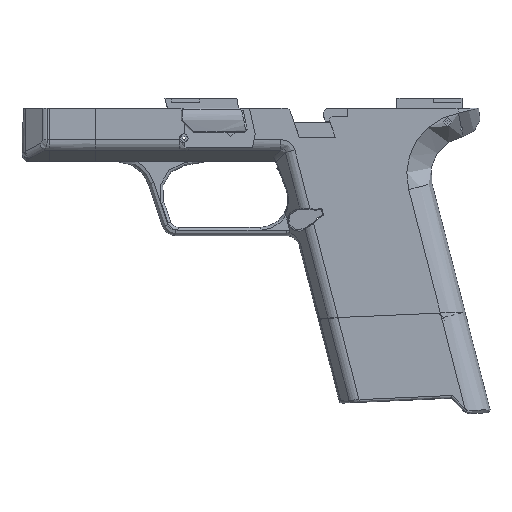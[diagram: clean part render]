
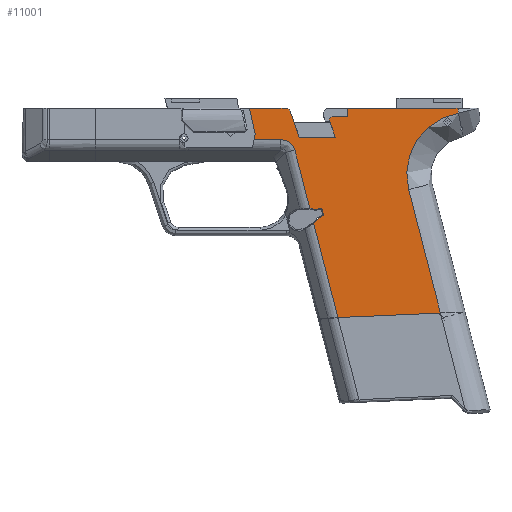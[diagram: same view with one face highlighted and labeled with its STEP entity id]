
A CAD part, left-side view. The second image highlights one B-rep face of the part: STEP entity #11001.
In plain terms, the highlighted face is planar.
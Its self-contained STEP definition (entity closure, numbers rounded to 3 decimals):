
#143=ELLIPSE('',#11910,10.693,7.);
#704=PLANE('',#11905);
#1143=FACE_OUTER_BOUND('',#1774,.T.);
#1774=EDGE_LOOP('',(#8642,#8643,#8644,#8645,#8646,#8647,#8648,#8649,#8650,
#8651,#8652,#8653,#8654,#8655,#8656,#8657,#8658,#8659,#8660,#8661,#8662,
#8663,#8664,#8665,#8666));
#2571=LINE('',#17867,#3620);
#2577=LINE('',#17877,#3626);
#2581=LINE('',#17885,#3630);
#2592=LINE('',#17944,#3641);
#2618=LINE('',#18009,#3667);
#2619=LINE('',#18011,#3668);
#2620=LINE('',#18013,#3669);
#2621=LINE('',#18019,#3670);
#2622=LINE('',#18021,#3671);
#2623=LINE('',#18023,#3672);
#2624=LINE('',#18027,#3673);
#2625=LINE('',#18029,#3674);
#2626=LINE('',#18031,#3675);
#2627=LINE('',#18035,#3676);
#2628=LINE('',#18037,#3677);
#2629=LINE('',#18039,#3678);
#2630=LINE('',#18041,#3679);
#2631=LINE('',#18044,#3680);
#3620=VECTOR('',#13763,10.);
#3626=VECTOR('',#13773,10.);
#3630=VECTOR('',#13781,10.);
#3641=VECTOR('',#13814,10.);
#3667=VECTOR('',#13874,10.);
#3668=VECTOR('',#13875,10.);
#3669=VECTOR('',#13876,10.);
#3670=VECTOR('',#13881,10.);
#3671=VECTOR('',#13882,10.);
#3672=VECTOR('',#13883,10.);
#3673=VECTOR('',#13886,10.);
#3674=VECTOR('',#13887,10.);
#3675=VECTOR('',#13888,10.);
#3676=VECTOR('',#13891,10.);
#3677=VECTOR('',#13892,10.);
#3678=VECTOR('',#13893,10.);
#3679=VECTOR('',#13894,10.);
#3680=VECTOR('',#13897,10.);
#4366=CIRCLE('',#11879,2.822);
#4367=CIRCLE('',#11883,2.822);
#4369=CIRCLE('',#11906,22.475);
#4370=CIRCLE('',#11907,7.5);
#4371=CIRCLE('',#11908,1.);
#4372=CIRCLE('',#11909,2.);
#4973=VERTEX_POINT('',#17864);
#4974=VERTEX_POINT('',#17866);
#4976=VERTEX_POINT('',#17875);
#4978=VERTEX_POINT('',#17884);
#4981=VERTEX_POINT('',#17898);
#4983=VERTEX_POINT('',#17905);
#4993=VERTEX_POINT('',#17942);
#5015=VERTEX_POINT('',#18008);
#5016=VERTEX_POINT('',#18010);
#5017=VERTEX_POINT('',#18012);
#5018=VERTEX_POINT('',#18014);
#5019=VERTEX_POINT('',#18016);
#5020=VERTEX_POINT('',#18018);
#5021=VERTEX_POINT('',#18020);
#5022=VERTEX_POINT('',#18022);
#5023=VERTEX_POINT('',#18024);
#5024=VERTEX_POINT('',#18026);
#5025=VERTEX_POINT('',#18028);
#5026=VERTEX_POINT('',#18030);
#5027=VERTEX_POINT('',#18032);
#5028=VERTEX_POINT('',#18034);
#5029=VERTEX_POINT('',#18036);
#5030=VERTEX_POINT('',#18038);
#5031=VERTEX_POINT('',#18040);
#5032=VERTEX_POINT('',#18042);
#6261=EDGE_CURVE('',#4974,#4973,#2571,.T.);
#6267=EDGE_CURVE('',#4973,#4976,#2577,.T.);
#6271=EDGE_CURVE('',#4978,#4974,#2581,.T.);
#6275=EDGE_CURVE('',#4976,#4981,#4366,.T.);
#6278=EDGE_CURVE('',#4983,#4978,#4367,.T.);
#6292=EDGE_CURVE('',#4981,#4993,#2592,.T.);
#6325=EDGE_CURVE('',#5015,#4993,#2618,.T.);
#6326=EDGE_CURVE('',#5016,#5015,#2619,.T.);
#6327=EDGE_CURVE('',#5017,#5016,#2620,.T.);
#6328=EDGE_CURVE('',#5018,#5017,#4369,.T.);
#6329=EDGE_CURVE('',#5019,#5018,#4370,.T.);
#6330=EDGE_CURVE('',#5019,#5020,#2621,.T.);
#6331=EDGE_CURVE('',#5020,#5021,#2622,.F.);
#6332=EDGE_CURVE('',#5021,#5022,#2623,.T.);
#6333=EDGE_CURVE('',#5023,#5022,#4371,.T.);
#6334=EDGE_CURVE('',#5023,#5024,#2624,.F.);
#6335=EDGE_CURVE('',#5024,#5025,#2625,.T.);
#6336=EDGE_CURVE('',#5025,#5026,#2626,.F.);
#6337=EDGE_CURVE('',#5027,#5026,#4372,.T.);
#6338=EDGE_CURVE('',#5027,#5028,#2627,.T.);
#6339=EDGE_CURVE('',#5028,#5029,#2628,.T.);
#6340=EDGE_CURVE('',#5029,#5030,#2629,.T.);
#6341=EDGE_CURVE('',#5031,#5030,#2630,.T.);
#6342=EDGE_CURVE('',#5032,#5031,#143,.T.);
#6343=EDGE_CURVE('',#4983,#5032,#2631,.T.);
#8642=ORIENTED_EDGE('',*,*,#6278,.T.);
#8643=ORIENTED_EDGE('',*,*,#6271,.T.);
#8644=ORIENTED_EDGE('',*,*,#6261,.T.);
#8645=ORIENTED_EDGE('',*,*,#6267,.T.);
#8646=ORIENTED_EDGE('',*,*,#6275,.T.);
#8647=ORIENTED_EDGE('',*,*,#6292,.T.);
#8648=ORIENTED_EDGE('',*,*,#6325,.F.);
#8649=ORIENTED_EDGE('',*,*,#6326,.F.);
#8650=ORIENTED_EDGE('',*,*,#6327,.F.);
#8651=ORIENTED_EDGE('',*,*,#6328,.F.);
#8652=ORIENTED_EDGE('',*,*,#6329,.F.);
#8653=ORIENTED_EDGE('',*,*,#6330,.T.);
#8654=ORIENTED_EDGE('',*,*,#6331,.T.);
#8655=ORIENTED_EDGE('',*,*,#6332,.T.);
#8656=ORIENTED_EDGE('',*,*,#6333,.F.);
#8657=ORIENTED_EDGE('',*,*,#6334,.T.);
#8658=ORIENTED_EDGE('',*,*,#6335,.T.);
#8659=ORIENTED_EDGE('',*,*,#6336,.T.);
#8660=ORIENTED_EDGE('',*,*,#6337,.F.);
#8661=ORIENTED_EDGE('',*,*,#6338,.T.);
#8662=ORIENTED_EDGE('',*,*,#6339,.T.);
#8663=ORIENTED_EDGE('',*,*,#6340,.T.);
#8664=ORIENTED_EDGE('',*,*,#6341,.F.);
#8665=ORIENTED_EDGE('',*,*,#6342,.F.);
#8666=ORIENTED_EDGE('',*,*,#6343,.F.);
#11001=ADVANCED_FACE('',(#1143),#704,.F.);
#11879=AXIS2_PLACEMENT_3D('',#17900,#13786,#13787);
#11883=AXIS2_PLACEMENT_3D('',#17906,#13794,#13795);
#11905=AXIS2_PLACEMENT_3D('',#18007,#13872,#13873);
#11906=AXIS2_PLACEMENT_3D('',#18015,#13877,#13878);
#11907=AXIS2_PLACEMENT_3D('',#18017,#13879,#13880);
#11908=AXIS2_PLACEMENT_3D('',#18025,#13884,#13885);
#11909=AXIS2_PLACEMENT_3D('',#18033,#13889,#13890);
#11910=AXIS2_PLACEMENT_3D('',#18043,#13895,#13896);
#13763=DIRECTION('',(0.,-0.323,0.947));
#13773=DIRECTION('',(0.,0.866,0.5));
#13781=DIRECTION('',(0.,-0.991,-0.133));
#13786=DIRECTION('center_axis',(-1.,0.,0.));
#13787=DIRECTION('ref_axis',(0.,-0.56,0.828));
#13794=DIRECTION('center_axis',(-1.,0.,0.));
#13795=DIRECTION('ref_axis',(0.,-0.504,-0.864));
#13814=DIRECTION('',(0.,0.828,0.56));
#13872=DIRECTION('center_axis',(-1.,0.,0.));
#13873=DIRECTION('ref_axis',(0.,1.,0.));
#13874=DIRECTION('',(0.,0.249,-0.969));
#13875=DIRECTION('',(0.,0.999,0.044));
#13876=DIRECTION('',(0.,-0.249,0.969));
#13877=DIRECTION('center_axis',(1.,0.,0.));
#13878=DIRECTION('ref_axis',(0.,0.,1.));
#13879=DIRECTION('center_axis',(1.,0.,0.));
#13880=DIRECTION('ref_axis',(0.,-0.97,-0.244));
#13881=DIRECTION('',(0.,1.,0.));
#13882=DIRECTION('',(0.,0.,-1.));
#13883=DIRECTION('',(0.,1.,0.));
#13884=DIRECTION('center_axis',(-1.,0.,0.));
#13885=DIRECTION('ref_axis',(0.,0.817,-0.576));
#13886=DIRECTION('',(0.,0.336,-0.942));
#13887=DIRECTION('',(0.,1.,0.));
#13888=DIRECTION('',(0.,-0.336,0.942));
#13889=DIRECTION('center_axis',(-1.,0.,0.));
#13890=DIRECTION('ref_axis',(0.,-0.576,-0.817));
#13891=DIRECTION('',(0.,1.,0.));
#13892=DIRECTION('',(0.,-0.21,0.978));
#13893=DIRECTION('',(0.,0.21,0.978));
#13894=DIRECTION('',(0.,1.,0.));
#13895=DIRECTION('center_axis',(1.,0.,0.));
#13896=DIRECTION('ref_axis',(0.,-0.714,-0.7));
#13897=DIRECTION('',(0.,0.249,-0.969));
#17864=CARTESIAN_POINT('',(22.175,-32.382,31.415));
#17866=CARTESIAN_POINT('',(22.175,-31.529,28.913));
#17867=CARTESIAN_POINT('',(22.175,-26.222,13.336));
#17875=CARTESIAN_POINT('',(22.175,-30.028,32.774));
#17877=CARTESIAN_POINT('',(22.175,-29.537,33.057));
#17884=CARTESIAN_POINT('',(22.175,-28.835,29.274));
#17885=CARTESIAN_POINT('',(22.175,-20.345,30.412));
#17898=CARTESIAN_POINT('',(22.175,-28.995,34.049));
#17900=CARTESIAN_POINT('Origin',(22.175,-27.413,31.712));
#17905=CARTESIAN_POINT('',(22.175,-27.244,28.895));
#17906=CARTESIAN_POINT('Origin',(22.175,-27.413,31.712));
#17942=CARTESIAN_POINT('',(22.175,-28.632,34.294));
#17944=CARTESIAN_POINT('',(22.175,-29.16,33.937));
#18007=CARTESIAN_POINT('Origin',(22.175,-7.921,2.186));
#18008=CARTESIAN_POINT('',(22.175,-37.447,68.587));
#18009=CARTESIAN_POINT('',(22.175,-26.659,26.619));
#18010=CARTESIAN_POINT('',(22.175,-74.722,66.935));
#18011=CARTESIAN_POINT('',(22.175,-40.785,68.439));
#18012=CARTESIAN_POINT('',(22.175,-63.184,22.049));
#18013=CARTESIAN_POINT('',(22.175,-75.103,68.418));
#18014=CARTESIAN_POINT('',(22.175,-81.332,-5.728));
#18015=CARTESIAN_POINT('Origin',(22.175,-84.951,16.453));
#18016=CARTESIAN_POINT('',(22.175,-81.106,-7.556));
#18017=CARTESIAN_POINT('Origin',(22.175,-88.606,-7.556));
#18018=CARTESIAN_POINT('',(22.175,-40.774,-7.556));
#18019=CARTESIAN_POINT('',(22.175,-84.951,-7.556));
#18020=CARTESIAN_POINT('',(22.175,-40.774,-4.331));
#18021=CARTESIAN_POINT('',(22.175,-40.774,-2.685));
#18022=CARTESIAN_POINT('',(22.175,-35.316,-4.331));
#18023=CARTESIAN_POINT('',(22.175,-20.598,-4.331));
#18024=CARTESIAN_POINT('',(22.175,-34.374,-2.995));
#18025=CARTESIAN_POINT('Origin',(22.175,-35.316,-3.331));
#18026=CARTESIAN_POINT('',(22.175,-36.514,3.));
#18027=CARTESIAN_POINT('',(22.175,-32.976,-6.913));
#18028=CARTESIAN_POINT('',(22.175,-23.407,3.));
#18029=CARTESIAN_POINT('',(22.175,-23.764,3.));
#18030=CARTESIAN_POINT('',(22.175,-20.114,-6.228));
#18031=CARTESIAN_POINT('',(22.175,-21.552,-2.199));
#18032=CARTESIAN_POINT('',(22.175,-18.23,-7.556));
#18033=CARTESIAN_POINT('Origin',(22.175,-18.23,-5.556));
#18034=CARTESIAN_POINT('',(22.175,-5.3,-7.556));
#18035=CARTESIAN_POINT('',(22.175,-86.951,-7.556));
#18036=CARTESIAN_POINT('',(22.175,-7.389,2.186));
#18037=CARTESIAN_POINT('',(22.175,-6.356,-2.63));
#18038=CARTESIAN_POINT('',(22.175,-7.025,3.884));
#18039=CARTESIAN_POINT('',(22.175,-7.4,2.132));
#18040=CARTESIAN_POINT('',(22.175,-16.536,3.884));
#18041=CARTESIAN_POINT('',(22.175,33.814,3.884));
#18042=CARTESIAN_POINT('',(22.175,-21.783,7.651));
#18043=CARTESIAN_POINT('Origin',(22.175,-12.907,12.884));
#18044=CARTESIAN_POINT('',(22.175,-26.659,26.619));
